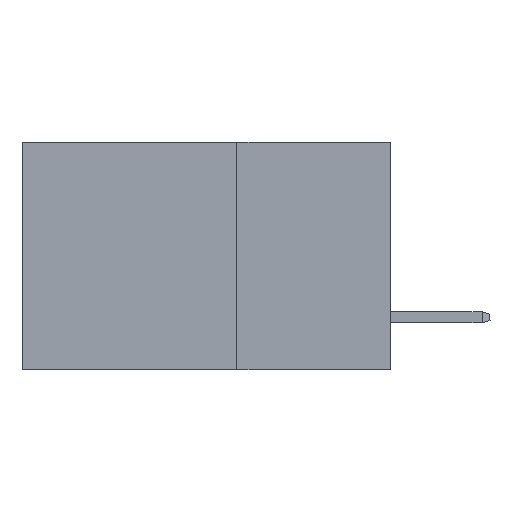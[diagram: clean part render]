
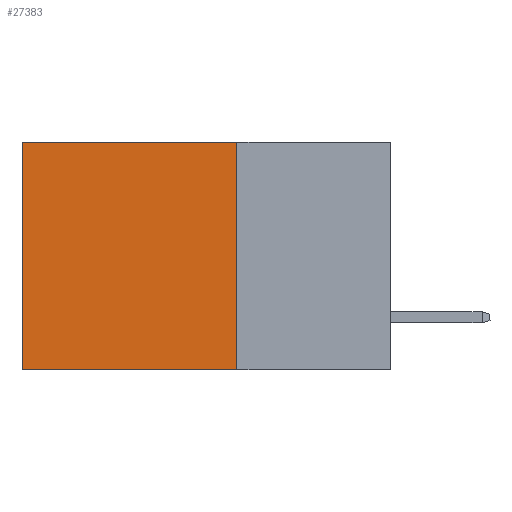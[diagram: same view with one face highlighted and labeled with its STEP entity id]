
A CAD part, left-side view. The second image highlights one B-rep face of the part: STEP entity #27383.
In plain terms, the highlighted planar face has unit normal (-1, 0, 0).
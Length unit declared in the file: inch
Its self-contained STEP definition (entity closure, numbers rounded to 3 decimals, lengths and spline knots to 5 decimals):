
#262 = VERTEX_POINT ( 'NONE', #30617 ) ;
#353 = DIRECTION ( 'NONE',  ( 0., 0., -1. ) ) ;
#1764 = LINE ( 'NONE', #2010, #20199 ) ;
#2010 = CARTESIAN_POINT ( 'NONE',  ( 0.2875, 0.25, 0. ) ) ;
#4432 = PLANE ( 'NONE',  #10904 ) ;
#4696 = VERTEX_POINT ( 'NONE', #29683 ) ;
#5067 = ORIENTED_EDGE ( 'NONE', *, *, #9819, .T. ) ;
#5207 = DIRECTION ( 'NONE',  ( 0., 0., -1. ) ) ;
#5728 = FACE_OUTER_BOUND ( 'NONE', #16639, .T. ) ;
#9819 = EDGE_CURVE ( 'NONE', #262, #4696, #22684, .T. ) ;
#9989 = CARTESIAN_POINT ( 'NONE',  ( 0.2875, 0.25, -0.37 ) ) ;
#10490 = VECTOR ( 'NONE', #17102, 39.37008 ) ;
#10904 = AXIS2_PLACEMENT_3D ( 'NONE', #26993, #12054, #29485 ) ;
#11559 = EDGE_CURVE ( 'NONE', #22341, #262, #1764, .T. ) ;
#12054 = DIRECTION ( 'NONE',  ( 1., 0., 0. ) ) ;
#14574 = CARTESIAN_POINT ( 'NONE',  ( 0.2875, 0.25, -0.37 ) ) ;
#14682 = ORIENTED_EDGE ( 'NONE', *, *, #11559, .T. ) ;
#15456 = VERTEX_POINT ( 'NONE', #9989 ) ;
#15882 = CARTESIAN_POINT ( 'NONE',  ( 0.2875, 0.25, 0. ) ) ;
#16639 = EDGE_LOOP ( 'NONE', ( #5067, #23908, #29670, #14682 ) ) ;
#17102 = DIRECTION ( 'NONE',  ( 0., 1., 0. ) ) ;
#18833 = VECTOR ( 'NONE', #353, 39.37008 ) ;
#19609 = LINE ( 'NONE', #27816, #18833 ) ;
#20199 = VECTOR ( 'NONE', #22068, 39.37008 ) ;
#20285 = EDGE_CURVE ( 'NONE', #22341, #15456, #19609, .T. ) ;
#21892 = VECTOR ( 'NONE', #5207, 39.37008 ) ;
#21976 = EDGE_CURVE ( 'NONE', #15456, #4696, #30330, .T. ) ;
#22068 = DIRECTION ( 'NONE',  ( 0., 1., 0. ) ) ;
#22341 = VERTEX_POINT ( 'NONE', #15882 ) ;
#22684 = LINE ( 'NONE', #27555, #21892 ) ;
#23908 = ORIENTED_EDGE ( 'NONE', *, *, #21976, .F. ) ;
#26993 = CARTESIAN_POINT ( 'NONE',  ( 0.2875, 0.25, 0. ) ) ;
#27383 = ADVANCED_FACE ( 'NONE', ( #5728 ), #4432, .F. ) ;
#27555 = CARTESIAN_POINT ( 'NONE',  ( 0.2875, 0.6, 0. ) ) ;
#27816 = CARTESIAN_POINT ( 'NONE',  ( 0.2875, 0.25, 0. ) ) ;
#29485 = DIRECTION ( 'NONE',  ( 0., 0., -1. ) ) ;
#29670 = ORIENTED_EDGE ( 'NONE', *, *, #20285, .F. ) ;
#29683 = CARTESIAN_POINT ( 'NONE',  ( 0.2875, 0.6, -0.37 ) ) ;
#30330 = LINE ( 'NONE', #14574, #10490 ) ;
#30617 = CARTESIAN_POINT ( 'NONE',  ( 0.2875, 0.6, 0. ) ) ;
